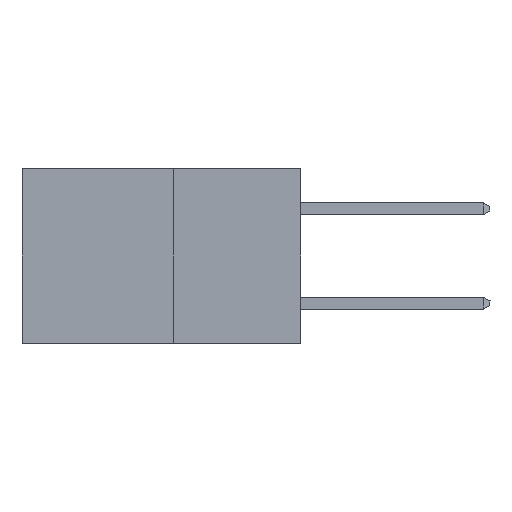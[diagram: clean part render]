
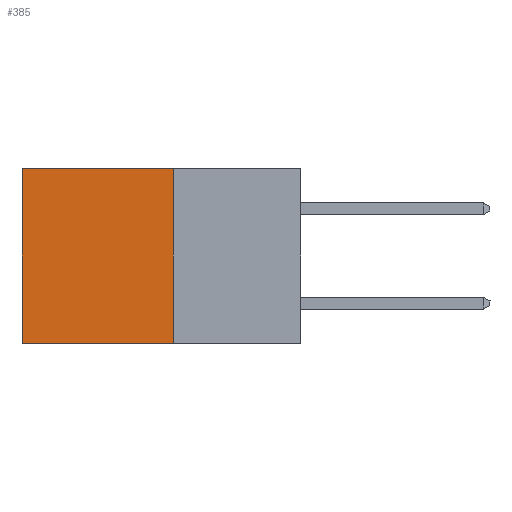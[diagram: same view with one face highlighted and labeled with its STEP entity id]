
A CAD part, left-side view. The second image highlights one B-rep face of the part: STEP entity #385.
In plain terms, the highlighted planar face has unit normal (-1, 0, 0).
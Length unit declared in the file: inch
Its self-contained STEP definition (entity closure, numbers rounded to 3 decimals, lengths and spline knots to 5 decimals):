
#346 = AXIS2_PLACEMENT_3D ( 'NONE', #2643, #4339, #493 ) ;
#385 = ADVANCED_FACE ( 'NONE', ( #8887 ), #3184, .F. ) ;
#493 = DIRECTION ( 'NONE',  ( 0., 0., -1. ) ) ;
#1019 = VERTEX_POINT ( 'NONE', #8069 ) ;
#1045 = EDGE_CURVE ( 'NONE', #1019, #5836, #4140, .T. ) ;
#1125 = ORIENTED_EDGE ( 'NONE', *, *, #2622, .F. ) ;
#1128 = LINE ( 'NONE', #1747, #2901 ) ;
#1328 = VECTOR ( 'NONE', #7671, 39.37008 ) ;
#1699 = VERTEX_POINT ( 'NONE', #5925 ) ;
#1716 = DIRECTION ( 'NONE',  ( 0., 1., 0. ) ) ;
#1747 = CARTESIAN_POINT ( 'NONE',  ( 0.277, 0.27, -0.37 ) ) ;
#2537 = EDGE_CURVE ( 'NONE', #5836, #1699, #8278, .T. ) ;
#2622 = EDGE_CURVE ( 'NONE', #8894, #1699, #1128, .T. ) ;
#2643 = CARTESIAN_POINT ( 'NONE',  ( 0.277, 0.27, -0.37 ) ) ;
#2746 = VECTOR ( 'NONE', #8728, 39.37008 ) ;
#2901 = VECTOR ( 'NONE', #1716, 39.37008 ) ;
#3184 = PLANE ( 'NONE',  #346 ) ;
#3614 = EDGE_CURVE ( 'NONE', #1019, #8894, #8482, .T. ) ;
#4021 = ORIENTED_EDGE ( 'NONE', *, *, #1045, .T. ) ;
#4140 = LINE ( 'NONE', #7986, #1328 ) ;
#4339 = DIRECTION ( 'NONE',  ( 1., 0., 0. ) ) ;
#4477 = CARTESIAN_POINT ( 'NONE',  ( 0.277, 0.59, 0. ) ) ;
#4634 = DIRECTION ( 'NONE',  ( 0., 0., -1. ) ) ;
#4790 = CARTESIAN_POINT ( 'NONE',  ( 0.277, 0.27, -0.37 ) ) ;
#5166 = CARTESIAN_POINT ( 'NONE',  ( 0.277, 0.59, -0.37 ) ) ;
#5836 = VERTEX_POINT ( 'NONE', #4477 ) ;
#5880 = ORIENTED_EDGE ( 'NONE', *, *, #2537, .T. ) ;
#5925 = CARTESIAN_POINT ( 'NONE',  ( 0.277, 0.59, -0.37 ) ) ;
#7671 = DIRECTION ( 'NONE',  ( 0., 1., 0. ) ) ;
#7986 = CARTESIAN_POINT ( 'NONE',  ( 0.277, 0.27, 0. ) ) ;
#8049 = VECTOR ( 'NONE', #4634, 39.37008 ) ;
#8069 = CARTESIAN_POINT ( 'NONE',  ( 0.277, 0.27, 0. ) ) ;
#8090 = ORIENTED_EDGE ( 'NONE', *, *, #3614, .F. ) ;
#8278 = LINE ( 'NONE', #5166, #8049 ) ;
#8482 = LINE ( 'NONE', #8842, #2746 ) ;
#8728 = DIRECTION ( 'NONE',  ( 0., 0., -1. ) ) ;
#8842 = CARTESIAN_POINT ( 'NONE',  ( 0.277, 0.27, -0.37 ) ) ;
#8887 = FACE_OUTER_BOUND ( 'NONE', #9537, .T. ) ;
#8894 = VERTEX_POINT ( 'NONE', #4790 ) ;
#9537 = EDGE_LOOP ( 'NONE', ( #5880, #1125, #8090, #4021 ) ) ;
